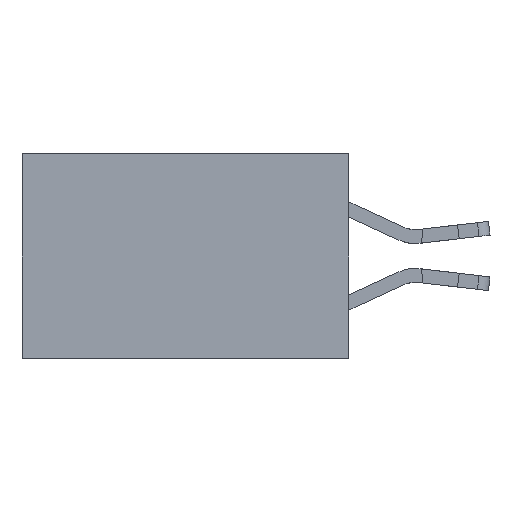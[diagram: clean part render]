
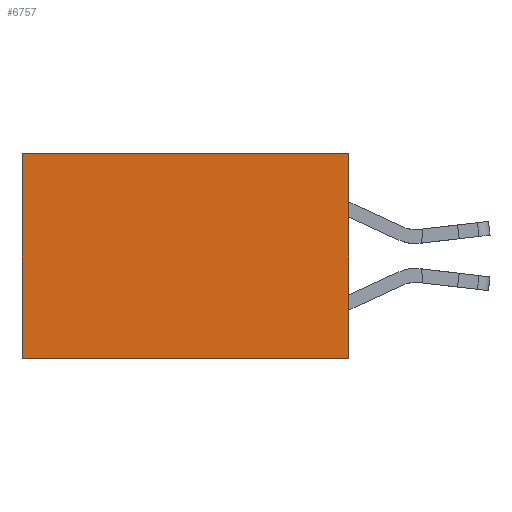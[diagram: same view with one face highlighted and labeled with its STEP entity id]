
A CAD part, left-side view. The second image highlights one B-rep face of the part: STEP entity #6757.
In plain terms, the highlighted planar face has unit normal (-1, 0, 0).
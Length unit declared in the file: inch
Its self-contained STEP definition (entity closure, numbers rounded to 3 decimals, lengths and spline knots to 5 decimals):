
#830 = DIRECTION ( 'NONE',  ( 0., 0., -1. ) ) ;
#886 = DIRECTION ( 'NONE',  ( 1., 0., 0. ) ) ;
#933 = PLANE ( 'NONE',  #18551 ) ;
#1183 = ORIENTED_EDGE ( 'NONE', *, *, #18499, .F. ) ;
#1439 = CARTESIAN_POINT ( 'NONE',  ( 0.277, 0., -0.37 ) ) ;
#3052 = DIRECTION ( 'NONE',  ( 0., 1., 0. ) ) ;
#3782 = CARTESIAN_POINT ( 'NONE',  ( 0.277, 0., -0.37 ) ) ;
#3787 = EDGE_CURVE ( 'NONE', #14500, #19484, #10115, .T. ) ;
#4716 = DIRECTION ( 'NONE',  ( 0., 0., -1. ) ) ;
#4923 = CARTESIAN_POINT ( 'NONE',  ( 0.277, 0., 0. ) ) ;
#5360 = ORIENTED_EDGE ( 'NONE', *, *, #3787, .T. ) ;
#5648 = VECTOR ( 'NONE', #14038, 39.37008 ) ;
#5906 = LINE ( 'NONE', #16460, #14422 ) ;
#5936 = CARTESIAN_POINT ( 'NONE',  ( 0.277, 0.59, -0.37 ) ) ;
#6757 = ADVANCED_FACE ( 'NONE', ( #14011 ), #933, .F. ) ;
#7976 = ORIENTED_EDGE ( 'NONE', *, *, #18693, .F. ) ;
#8470 = CARTESIAN_POINT ( 'NONE',  ( 0.277, 0.59, 0. ) ) ;
#9962 = VECTOR ( 'NONE', #3052, 39.37008 ) ;
#10115 = LINE ( 'NONE', #16675, #14086 ) ;
#10259 = CARTESIAN_POINT ( 'NONE',  ( 0.277, 0., -0.37 ) ) ;
#10492 = LINE ( 'NONE', #20375, #9962 ) ;
#12737 = VERTEX_POINT ( 'NONE', #10259 ) ;
#14011 = FACE_OUTER_BOUND ( 'NONE', #20949, .T. ) ;
#14038 = DIRECTION ( 'NONE',  ( 0., 0., -1. ) ) ;
#14086 = VECTOR ( 'NONE', #4716, 39.37008 ) ;
#14422 = VECTOR ( 'NONE', #18228, 39.37008 ) ;
#14500 = VERTEX_POINT ( 'NONE', #8470 ) ;
#15058 = VERTEX_POINT ( 'NONE', #4923 ) ;
#15232 = LINE ( 'NONE', #3782, #5648 ) ;
#16460 = CARTESIAN_POINT ( 'NONE',  ( 0.277, 0., 0. ) ) ;
#16675 = CARTESIAN_POINT ( 'NONE',  ( 0.277, 0.59, -0.37 ) ) ;
#18228 = DIRECTION ( 'NONE',  ( 0., 1., 0. ) ) ;
#18499 = EDGE_CURVE ( 'NONE', #12737, #19484, #10492, .T. ) ;
#18551 = AXIS2_PLACEMENT_3D ( 'NONE', #1439, #886, #830 ) ;
#18693 = EDGE_CURVE ( 'NONE', #15058, #12737, #15232, .T. ) ;
#19400 = ORIENTED_EDGE ( 'NONE', *, *, #20791, .T. ) ;
#19484 = VERTEX_POINT ( 'NONE', #5936 ) ;
#20375 = CARTESIAN_POINT ( 'NONE',  ( 0.277, 0., -0.37 ) ) ;
#20791 = EDGE_CURVE ( 'NONE', #15058, #14500, #5906, .T. ) ;
#20949 = EDGE_LOOP ( 'NONE', ( #5360, #1183, #7976, #19400 ) ) ;
